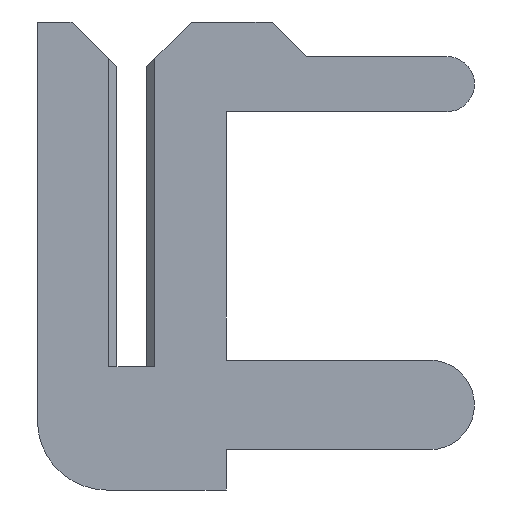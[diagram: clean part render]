
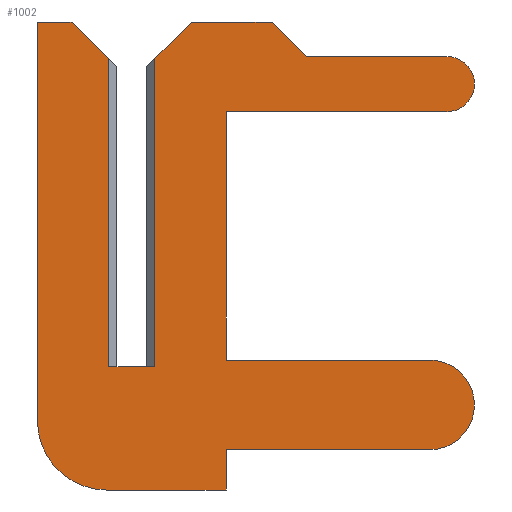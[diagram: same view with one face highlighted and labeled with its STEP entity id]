
A CAD part, left-side view. The second image highlights one B-rep face of the part: STEP entity #1002.
In plain terms, the highlighted planar face has unit normal (-1, 0, 0).
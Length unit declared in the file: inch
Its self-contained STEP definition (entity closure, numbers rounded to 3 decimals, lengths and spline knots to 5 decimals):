
#3 = CARTESIAN_POINT ( 'NONE',  ( -0.01, -0.076, 0.135 ) ) ;
#8 = CIRCLE ( 'NONE', #49, 0.012 ) ;
#12 = PLANE ( 'NONE',  #888 ) ;
#20 = VECTOR ( 'NONE', #779, 39.37008 ) ;
#25 = ORIENTED_EDGE ( 'NONE', *, *, #100, .F. ) ;
#29 = CARTESIAN_POINT ( 'NONE',  ( -0.01, 0.0065, 0.1305 ) ) ;
#32 = CARTESIAN_POINT ( 'NONE',  ( -0.01, 0.041, -0.0235 ) ) ;
#45 = LINE ( 'NONE', #177, #117 ) ;
#48 = VERTEX_POINT ( 'NONE', #287 ) ;
#49 = AXIS2_PLACEMENT_3D ( 'NONE', #471, #696, #129 ) ;
#56 = VECTOR ( 'NONE', #404, 39.37008 ) ;
#75 = LINE ( 'NONE', #734, #541 ) ;
#79 = CARTESIAN_POINT ( 'NONE',  ( -0.01, 0.011, -0.0535 ) ) ;
#90 = DIRECTION ( 'NONE',  ( -1., 0., 0. ) ) ;
#95 = DIRECTION ( 'NONE',  ( 0., -1., 0. ) ) ;
#96 = VERTEX_POINT ( 'NONE', #32 ) ;
#99 = EDGE_CURVE ( 'NONE', #714, #96, #178, .T. ) ;
#100 = EDGE_CURVE ( 'NONE', #132, #793, #8, .T. ) ;
#102 = DIRECTION ( 'NONE',  ( 0., -1., 0. ) ) ;
#117 = VECTOR ( 'NONE', #737, 39.37008 ) ;
#123 = ORIENTED_EDGE ( 'NONE', *, *, #595, .F. ) ;
#127 = DIRECTION ( 'NONE',  ( 0., 0., 1. ) ) ;
#129 = DIRECTION ( 'NONE',  ( 0., 0., 1. ) ) ;
#132 = VERTEX_POINT ( 'NONE', #377 ) ;
#134 = VERTEX_POINT ( 'NONE', #224 ) ;
#154 = CARTESIAN_POINT ( 'NONE',  ( -0.01, 0.01, 0.134 ) ) ;
#162 = ORIENTED_EDGE ( 'NONE', *, *, #324, .F. ) ;
#166 = EDGE_CURVE ( 'NONE', #965, #914, #451, .T. ) ;
#177 = CARTESIAN_POINT ( 'NONE',  ( -0.01, -0.076, 0.135 ) ) ;
#178 = CIRCLE ( 'NONE', #740, 0.03 ) ;
#179 = VERTEX_POINT ( 'NONE', #1010 ) ;
#182 = CARTESIAN_POINT ( 'NONE',  ( -0.01, 0.026, 0.15 ) ) ;
#186 = CARTESIAN_POINT ( 'NONE',  ( -0.01, 0.01, -0.0235 ) ) ;
#189 = EDGE_CURVE ( 'NONE', #793, #965, #789, .T. ) ;
#199 = VECTOR ( 'NONE', #102, 39.37008 ) ;
#217 = ORIENTED_EDGE ( 'NONE', *, *, #356, .F. ) ;
#219 = CARTESIAN_POINT ( 'NONE',  ( -0.01, 0.011, -0.0235 ) ) ;
#224 = CARTESIAN_POINT ( 'NONE',  ( -0.01, -0.041, -0.0535 ) ) ;
#251 = EDGE_LOOP ( 'NONE', ( #978, #531, #123, #544, #429, #849, #533, #713, #607, #935, #803, #794, #162, #694, #413, #25, #217, #1018, #715 ) ) ;
#252 = VERTEX_POINT ( 'NONE', #560 ) ;
#258 = DIRECTION ( 'NONE',  ( 0., 0., -1. ) ) ;
#270 = CARTESIAN_POINT ( 'NONE',  ( -0.01, -0.01, 0.15 ) ) ;
#272 = AXIS2_PLACEMENT_3D ( 'NONE', #315, #948, #797 ) ;
#274 = FACE_OUTER_BOUND ( 'NONE', #251, .T. ) ;
#283 = VECTOR ( 'NONE', #95, 39.37008 ) ;
#287 = CARTESIAN_POINT ( 'NONE',  ( -0.01, -0.061, 0.15 ) ) ;
#294 = LINE ( 'NONE', #877, #701 ) ;
#298 = DIRECTION ( 'NONE',  ( 1., 0., 0. ) ) ;
#302 = CARTESIAN_POINT ( 'NONE',  ( -0.01, -0.041, 0.003 ) ) ;
#315 = CARTESIAN_POINT ( 'NONE',  ( -0.01, -0.1295, -0.0165 ) ) ;
#317 = CARTESIAN_POINT ( 'NONE',  ( -0.01, -0.137, 0.135 ) ) ;
#320 = VECTOR ( 'NONE', #258, 39.37008 ) ;
#324 = EDGE_CURVE ( 'NONE', #914, #179, #838, .T. ) ;
#331 = CARTESIAN_POINT ( 'NONE',  ( -0.01, 0.011, -0.0235 ) ) ;
#332 = LINE ( 'NONE', #270, #320 ) ;
#356 = EDGE_CURVE ( 'NONE', #569, #132, #933, .T. ) ;
#358 = VECTOR ( 'NONE', #633, 39.37008 ) ;
#362 = DIRECTION ( 'NONE',  ( 0., -0.707, -0.707 ) ) ;
#367 = LINE ( 'NONE', #596, #56 ) ;
#368 = EDGE_CURVE ( 'NONE', #771, #134, #294, .T. ) ;
#373 = VERTEX_POINT ( 'NONE', #402 ) ;
#375 = EDGE_CURVE ( 'NONE', #885, #771, #553, .T. ) ;
#377 = CARTESIAN_POINT ( 'NONE',  ( -0.01, -0.137, 0.135 ) ) ;
#392 = CARTESIAN_POINT ( 'NONE',  ( -0.01, 0.041, 0.15 ) ) ;
#402 = CARTESIAN_POINT ( 'NONE',  ( -0.01, 0.026, 0.15 ) ) ;
#404 = DIRECTION ( 'NONE',  ( 0., -1., 0. ) ) ;
#413 = ORIENTED_EDGE ( 'NONE', *, *, #189, .F. ) ;
#429 = ORIENTED_EDGE ( 'NONE', *, *, #545, .F. ) ;
#449 = EDGE_CURVE ( 'NONE', #48, #569, #45, .T. ) ;
#451 = LINE ( 'NONE', #302, #20 ) ;
#470 = EDGE_CURVE ( 'NONE', #832, #373, #973, .T. ) ;
#471 = CARTESIAN_POINT ( 'NONE',  ( -0.01, -0.137, 0.123 ) ) ;
#473 = DIRECTION ( 'NONE',  ( 0., 0., -1. ) ) ;
#482 = CARTESIAN_POINT ( 'NONE',  ( -0.01, -0.137, 0.111 ) ) ;
#483 = VECTOR ( 'NONE', #841, 39.37008 ) ;
#498 = CARTESIAN_POINT ( 'NONE',  ( -0.01, -0.026, 0.15 ) ) ;
#531 = ORIENTED_EDGE ( 'NONE', *, *, #592, .T. ) ;
#533 = ORIENTED_EDGE ( 'NONE', *, *, #678, .F. ) ;
#537 = DIRECTION ( 'NONE',  ( 0., 1., 0. ) ) ;
#541 = VECTOR ( 'NONE', #572, 39.37008 ) ;
#544 = ORIENTED_EDGE ( 'NONE', *, *, #1025, .T. ) ;
#545 = EDGE_CURVE ( 'NONE', #373, #963, #864, .T. ) ;
#553 = LINE ( 'NONE', #1016, #358 ) ;
#560 = CARTESIAN_POINT ( 'NONE',  ( -0.01, 0.01, 0. ) ) ;
#561 = CARTESIAN_POINT ( 'NONE',  ( -0.01, -0.041, 0.003 ) ) ;
#569 = VERTEX_POINT ( 'NONE', #3 ) ;
#572 = DIRECTION ( 'NONE',  ( 0., -0.707, 0.707 ) ) ;
#576 = EDGE_CURVE ( 'NONE', #943, #48, #367, .T. ) ;
#587 = DIRECTION ( 'NONE',  ( 0., 0., 1. ) ) ;
#592 = EDGE_CURVE ( 'NONE', #805, #875, #332, .T. ) ;
#595 = EDGE_CURVE ( 'NONE', #252, #875, #725, .T. ) ;
#596 = CARTESIAN_POINT ( 'NONE',  ( -0.01, -0.026, 0.15 ) ) ;
#607 = ORIENTED_EDGE ( 'NONE', *, *, #863, .F. ) ;
#623 = LINE ( 'NONE', #79, #972 ) ;
#631 = DIRECTION ( 'NONE',  ( 0., -1., 0. ) ) ;
#633 = DIRECTION ( 'NONE',  ( 0., 1., 0. ) ) ;
#636 = CARTESIAN_POINT ( 'NONE',  ( -0.01, -0.1295, 0.003 ) ) ;
#638 = LINE ( 'NONE', #186, #675 ) ;
#646 = CARTESIAN_POINT ( 'NONE',  ( -0.01, -0.041, -0.036 ) ) ;
#670 = CARTESIAN_POINT ( 'NONE',  ( -0.01, -0.041, 0.111 ) ) ;
#675 = VECTOR ( 'NONE', #747, 39.37008 ) ;
#678 = EDGE_CURVE ( 'NONE', #96, #832, #990, .T. ) ;
#686 = EDGE_CURVE ( 'NONE', #179, #885, #862, .T. ) ;
#694 = ORIENTED_EDGE ( 'NONE', *, *, #166, .F. ) ;
#696 = DIRECTION ( 'NONE',  ( 1., 0., 0. ) ) ;
#701 = VECTOR ( 'NONE', #473, 39.37008 ) ;
#713 = ORIENTED_EDGE ( 'NONE', *, *, #99, .F. ) ;
#714 = VERTEX_POINT ( 'NONE', #772 ) ;
#715 = ORIENTED_EDGE ( 'NONE', *, *, #576, .F. ) ;
#719 = DIRECTION ( 'NONE',  ( 0., 1., 0. ) ) ;
#724 = CARTESIAN_POINT ( 'NONE',  ( -0.01, -0.01, 0.134 ) ) ;
#725 = LINE ( 'NONE', #824, #199 ) ;
#726 = VECTOR ( 'NONE', #631, 39.37008 ) ;
#734 = CARTESIAN_POINT ( 'NONE',  ( -0.01, -0.0065, 0.1305 ) ) ;
#737 = DIRECTION ( 'NONE',  ( 0., -0.707, -0.707 ) ) ;
#740 = AXIS2_PLACEMENT_3D ( 'NONE', #219, #298, #127 ) ;
#742 = VECTOR ( 'NONE', #886, 39.37008 ) ;
#747 = DIRECTION ( 'NONE',  ( 0., 0., 1. ) ) ;
#756 = VECTOR ( 'NONE', #362, 39.37008 ) ;
#766 = VECTOR ( 'NONE', #537, 39.37008 ) ;
#771 = VERTEX_POINT ( 'NONE', #646 ) ;
#772 = CARTESIAN_POINT ( 'NONE',  ( -0.01, 0.011, -0.0535 ) ) ;
#779 = DIRECTION ( 'NONE',  ( 0., 0., -1. ) ) ;
#789 = LINE ( 'NONE', #1006, #766 ) ;
#793 = VERTEX_POINT ( 'NONE', #482 ) ;
#794 = ORIENTED_EDGE ( 'NONE', *, *, #686, .F. ) ;
#797 = DIRECTION ( 'NONE',  ( 0., 0., 1. ) ) ;
#803 = ORIENTED_EDGE ( 'NONE', *, *, #375, .F. ) ;
#805 = VERTEX_POINT ( 'NONE', #724 ) ;
#824 = CARTESIAN_POINT ( 'NONE',  ( -0.01, 0.0065, 0. ) ) ;
#832 = VERTEX_POINT ( 'NONE', #392 ) ;
#838 = LINE ( 'NONE', #636, #726 ) ;
#841 = DIRECTION ( 'NONE',  ( 0., 0., 1. ) ) ;
#847 = CARTESIAN_POINT ( 'NONE',  ( -0.01, 0.041, 0.15 ) ) ;
#848 = EDGE_CURVE ( 'NONE', #805, #943, #75, .T. ) ;
#849 = ORIENTED_EDGE ( 'NONE', *, *, #470, .F. ) ;
#862 = CIRCLE ( 'NONE', #272, 0.0195 ) ;
#863 = EDGE_CURVE ( 'NONE', #134, #714, #623, .T. ) ;
#864 = LINE ( 'NONE', #29, #756 ) ;
#875 = VERTEX_POINT ( 'NONE', #956 ) ;
#877 = CARTESIAN_POINT ( 'NONE',  ( -0.01, -0.041, -0.0535 ) ) ;
#885 = VERTEX_POINT ( 'NONE', #1029 ) ;
#886 = DIRECTION ( 'NONE',  ( 0., -1., 0. ) ) ;
#888 = AXIS2_PLACEMENT_3D ( 'NONE', #331, #90, #587 ) ;
#914 = VERTEX_POINT ( 'NONE', #561 ) ;
#933 = LINE ( 'NONE', #317, #742 ) ;
#935 = ORIENTED_EDGE ( 'NONE', *, *, #368, .F. ) ;
#943 = VERTEX_POINT ( 'NONE', #498 ) ;
#948 = DIRECTION ( 'NONE',  ( 1., 0., 0. ) ) ;
#956 = CARTESIAN_POINT ( 'NONE',  ( -0.01, -0.01, 0. ) ) ;
#963 = VERTEX_POINT ( 'NONE', #154 ) ;
#965 = VERTEX_POINT ( 'NONE', #670 ) ;
#972 = VECTOR ( 'NONE', #719, 39.37008 ) ;
#973 = LINE ( 'NONE', #182, #283 ) ;
#978 = ORIENTED_EDGE ( 'NONE', *, *, #848, .F. ) ;
#990 = LINE ( 'NONE', #847, #483 ) ;
#1002 = ADVANCED_FACE ( 'NONE', ( #274 ), #12, .T. ) ;
#1006 = CARTESIAN_POINT ( 'NONE',  ( -0.01, -0.041, 0.111 ) ) ;
#1010 = CARTESIAN_POINT ( 'NONE',  ( -0.01, -0.1295, 0.003 ) ) ;
#1016 = CARTESIAN_POINT ( 'NONE',  ( -0.01, -0.041, -0.036 ) ) ;
#1018 = ORIENTED_EDGE ( 'NONE', *, *, #449, .F. ) ;
#1025 = EDGE_CURVE ( 'NONE', #252, #963, #638, .T. ) ;
#1029 = CARTESIAN_POINT ( 'NONE',  ( -0.01, -0.1295, -0.036 ) ) ;
